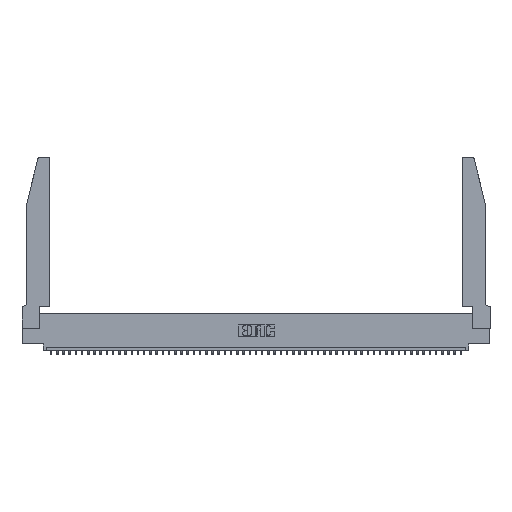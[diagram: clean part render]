
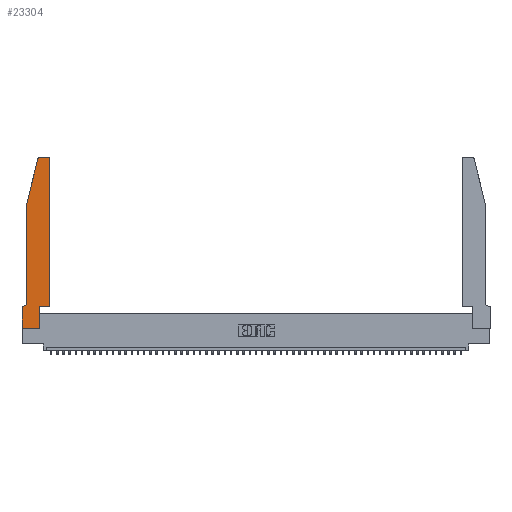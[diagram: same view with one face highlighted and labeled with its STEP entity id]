
A CAD part, top view. The second image highlights one B-rep face of the part: STEP entity #23304.
In plain terms, the highlighted planar face has unit normal (0, 0, 1).
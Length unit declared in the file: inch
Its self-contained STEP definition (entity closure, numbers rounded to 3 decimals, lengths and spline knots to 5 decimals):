
#792 = LINE ( 'NONE', #805, #6551 ) ;
#805 = CARTESIAN_POINT ( 'NONE',  ( 0.4505, 0.35, 0.37 ) ) ;
#872 = EDGE_CURVE ( 'NONE', #20992, #43772, #4781, .T. ) ;
#1248 = ORIENTED_EDGE ( 'NONE', *, *, #24904, .T. ) ;
#1337 = VECTOR ( 'NONE', #7828, 39.37008 ) ;
#1397 = VERTEX_POINT ( 'NONE', #12611 ) ;
#2461 = CIRCLE ( 'NONE', #5274, 0.03 ) ;
#4774 = CARTESIAN_POINT ( 'NONE',  ( 0.4205, 2.72, 0.37 ) ) ;
#4781 = LINE ( 'NONE', #7917, #44954 ) ;
#5274 = AXIS2_PLACEMENT_3D ( 'NONE', #4774, #33004, #49190 ) ;
#5496 = CARTESIAN_POINT ( 'NONE',  ( 0.0055, 0.42, 0.37 ) ) ;
#5726 = LINE ( 'NONE', #15483, #47322 ) ;
#6039 = EDGE_CURVE ( 'NONE', #9879, #32709, #792, .T. ) ;
#6518 = LINE ( 'NONE', #47207, #1337 ) ;
#6551 = VECTOR ( 'NONE', #9450, 39.37008 ) ;
#7828 = DIRECTION ( 'NONE',  ( -1., 0., 0. ) ) ;
#7879 = CARTESIAN_POINT ( 'NONE',  ( 0.284, 2.72, 0.37 ) ) ;
#7917 = CARTESIAN_POINT ( 'NONE',  ( 0.2605, 2.75, 0.37 ) ) ;
#8571 = EDGE_CURVE ( 'NONE', #38225, #19100, #49771, .T. ) ;
#8777 = EDGE_LOOP ( 'NONE', ( #43616, #51628, #19967, #1248, #38219, #21276, #25583, #19830, #12696, #36345, #26833, #17269 ) ) ;
#9325 = DIRECTION ( 'NONE',  ( 0., -1., 0. ) ) ;
#9450 = DIRECTION ( 'NONE',  ( 1., 0., 0. ) ) ;
#9744 = CARTESIAN_POINT ( 'NONE',  ( 0.0055, 0.35, 0.37 ) ) ;
#9879 = VERTEX_POINT ( 'NONE', #26717 ) ;
#10076 = EDGE_CURVE ( 'NONE', #19100, #23936, #40076, .T. ) ;
#10781 = VECTOR ( 'NONE', #24095, 39.37008 ) ;
#11936 = DIRECTION ( 'NONE',  ( -1., 0., 0. ) ) ;
#12611 = CARTESIAN_POINT ( 'NONE',  ( 0.0755, 0.42, 0.37 ) ) ;
#12696 = ORIENTED_EDGE ( 'NONE', *, *, #26910, .T. ) ;
#13565 = DIRECTION ( 'NONE',  ( 0., 0., -1. ) ) ;
#14720 = LINE ( 'NONE', #29293, #10781 ) ;
#15124 = DIRECTION ( 'NONE',  ( 0., 1., 0. ) ) ;
#15427 = DIRECTION ( 'NONE',  ( 0., 0., 1. ) ) ;
#15483 = CARTESIAN_POINT ( 'NONE',  ( 0.4505, 0.35, 0.37 ) ) ;
#15582 = VERTEX_POINT ( 'NONE', #18932 ) ;
#16187 = CARTESIAN_POINT ( 'NONE',  ( 0., 0.35, 0.37 ) ) ;
#16808 = CARTESIAN_POINT ( 'NONE',  ( 0.2865, 0., 0.37 ) ) ;
#17269 = ORIENTED_EDGE ( 'NONE', *, *, #20914, .T. ) ;
#18932 = CARTESIAN_POINT ( 'NONE',  ( 0.0755, 2., 0.37 ) ) ;
#18993 = VERTEX_POINT ( 'NONE', #38909 ) ;
#19039 = DIRECTION ( 'NONE',  ( 1., 0., 0. ) ) ;
#19100 = VERTEX_POINT ( 'NONE', #30359 ) ;
#19830 = ORIENTED_EDGE ( 'NONE', *, *, #10076, .T. ) ;
#19967 = ORIENTED_EDGE ( 'NONE', *, *, #51274, .T. ) ;
#20369 = DIRECTION ( 'NONE',  ( 0., 0., 1. ) ) ;
#20914 = EDGE_CURVE ( 'NONE', #18993, #20992, #2461, .T. ) ;
#20992 = VERTEX_POINT ( 'NONE', #46233 ) ;
#21085 = CARTESIAN_POINT ( 'NONE',  ( 0.4505, 0.35, 0.37 ) ) ;
#21156 = VECTOR ( 'NONE', #25567, 39.37008 ) ;
#21276 = ORIENTED_EDGE ( 'NONE', *, *, #26860, .T. ) ;
#22480 = LINE ( 'NONE', #45583, #21156 ) ;
#23304 = ADVANCED_FACE ( 'NONE', ( #45542 ), #45505, .T. ) ;
#23931 = AXIS2_PLACEMENT_3D ( 'NONE', #5496, #13565, #41654 ) ;
#23936 = VERTEX_POINT ( 'NONE', #16808 ) ;
#23993 = VERTEX_POINT ( 'NONE', #9744 ) ;
#24095 = DIRECTION ( 'NONE',  ( 0., 1., 0. ) ) ;
#24904 = EDGE_CURVE ( 'NONE', #15582, #1397, #43567, .T. ) ;
#25271 = CARTESIAN_POINT ( 'NONE',  ( 0., 0., 0.37 ) ) ;
#25567 = DIRECTION ( 'NONE',  ( -0.239, -0.971, 0. ) ) ;
#25583 = ORIENTED_EDGE ( 'NONE', *, *, #8571, .T. ) ;
#26717 = CARTESIAN_POINT ( 'NONE',  ( 0.2865, 0.35, 0.37 ) ) ;
#26833 = ORIENTED_EDGE ( 'NONE', *, *, #34643, .T. ) ;
#26860 = EDGE_CURVE ( 'NONE', #23993, #38225, #6518, .T. ) ;
#26910 = EDGE_CURVE ( 'NONE', #23936, #9879, #14720, .T. ) ;
#27391 = DIRECTION ( 'NONE',  ( 1., 0., 0. ) ) ;
#29293 = CARTESIAN_POINT ( 'NONE',  ( 0.2865, 0.35, 0.37 ) ) ;
#29920 = CIRCLE ( 'NONE', #23931, 0.07 ) ;
#30359 = CARTESIAN_POINT ( 'NONE',  ( 0., 0., 0.37 ) ) ;
#32059 = AXIS2_PLACEMENT_3D ( 'NONE', #16187, #20369, #40583 ) ;
#32238 = CARTESIAN_POINT ( 'NONE',  ( 0.25487, 2.72718, 0.37 ) ) ;
#32709 = VERTEX_POINT ( 'NONE', #21085 ) ;
#33004 = DIRECTION ( 'NONE',  ( 0., 0., 1. ) ) ;
#33924 = EDGE_CURVE ( 'NONE', #43772, #42291, #41583, .T. ) ;
#34307 = AXIS2_PLACEMENT_3D ( 'NONE', #7879, #15427, #27391 ) ;
#34643 = EDGE_CURVE ( 'NONE', #32709, #18993, #5726, .T. ) ;
#36345 = ORIENTED_EDGE ( 'NONE', *, *, #6039, .T. ) ;
#37498 = VECTOR ( 'NONE', #19039, 39.37008 ) ;
#38153 = CARTESIAN_POINT ( 'NONE',  ( 0.284, 2.75, 0.37 ) ) ;
#38219 = ORIENTED_EDGE ( 'NONE', *, *, #44706, .T. ) ;
#38225 = VERTEX_POINT ( 'NONE', #41122 ) ;
#38909 = CARTESIAN_POINT ( 'NONE',  ( 0.4505, 2.72, 0.37 ) ) ;
#40076 = LINE ( 'NONE', #40330, #37498 ) ;
#40292 = CARTESIAN_POINT ( 'NONE',  ( 0.0755, 2., 0.37 ) ) ;
#40330 = CARTESIAN_POINT ( 'NONE',  ( 0., 0., 0.37 ) ) ;
#40583 = DIRECTION ( 'NONE',  ( 1., 0., 0. ) ) ;
#41122 = CARTESIAN_POINT ( 'NONE',  ( 0., 0.35, 0.37 ) ) ;
#41583 = CIRCLE ( 'NONE', #34307, 0.03 ) ;
#41654 = DIRECTION ( 'NONE',  ( -1., 0., 0. ) ) ;
#42291 = VERTEX_POINT ( 'NONE', #32238 ) ;
#43567 = LINE ( 'NONE', #40292, #46030 ) ;
#43616 = ORIENTED_EDGE ( 'NONE', *, *, #872, .T. ) ;
#43772 = VERTEX_POINT ( 'NONE', #38153 ) ;
#44706 = EDGE_CURVE ( 'NONE', #1397, #23993, #29920, .T. ) ;
#44954 = VECTOR ( 'NONE', #11936, 39.37008 ) ;
#45505 = PLANE ( 'NONE',  #32059 ) ;
#45542 = FACE_OUTER_BOUND ( 'NONE', #8777, .T. ) ;
#45583 = CARTESIAN_POINT ( 'NONE',  ( 0.0755, 2., 0.37 ) ) ;
#46030 = VECTOR ( 'NONE', #48408, 39.37008 ) ;
#46233 = CARTESIAN_POINT ( 'NONE',  ( 0.4205, 2.75, 0.37 ) ) ;
#47207 = CARTESIAN_POINT ( 'NONE',  ( 0.0755, 0.35, 0.37 ) ) ;
#47322 = VECTOR ( 'NONE', #15124, 39.37008 ) ;
#47372 = VECTOR ( 'NONE', #9325, 39.37008 ) ;
#48408 = DIRECTION ( 'NONE',  ( 0., -1., 0. ) ) ;
#49190 = DIRECTION ( 'NONE',  ( 1., 0., 0. ) ) ;
#49771 = LINE ( 'NONE', #25271, #47372 ) ;
#51274 = EDGE_CURVE ( 'NONE', #42291, #15582, #22480, .T. ) ;
#51628 = ORIENTED_EDGE ( 'NONE', *, *, #33924, .T. ) ;
